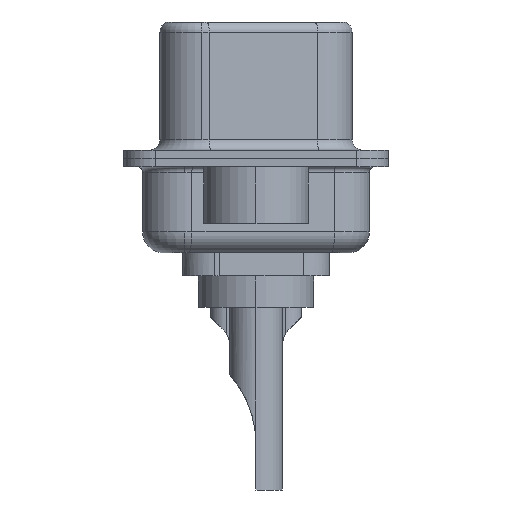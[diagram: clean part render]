
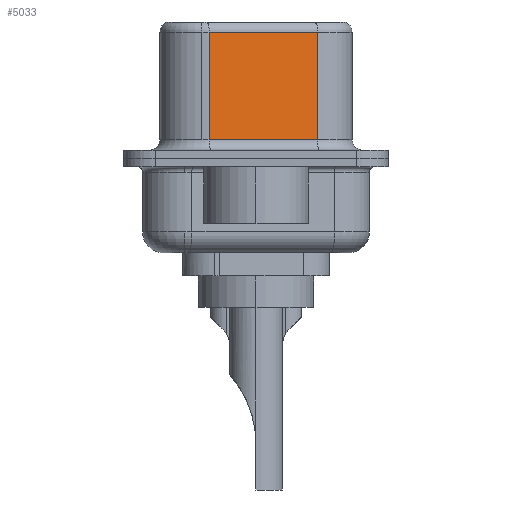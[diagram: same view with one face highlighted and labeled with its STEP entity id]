
A CAD part, left-side view. The second image highlights one B-rep face of the part: STEP entity #5033.
In plain terms, the highlighted planar face has unit normal (-0.985, -0.174, 0).
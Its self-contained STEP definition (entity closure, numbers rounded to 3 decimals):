
#11 = CARTESIAN_POINT ( 'NONE',  ( 4.585, -2.927, 0.9 ) ) ;
#1015 = VERTEX_POINT ( 'NONE', #20164 ) ;
#1697 = AXIS2_PLACEMENT_3D ( 'NONE', #19603, #19473, #19910 ) ;
#2051 = ORIENTED_EDGE ( 'NONE', *, *, #18329, .T. ) ;
#3246 = LINE ( 'NONE', #13953, #20159 ) ;
#4359 = DIRECTION ( 'NONE',  ( 0., 0., -1. ) ) ;
#5033 = ADVANCED_FACE ( 'NONE', ( #6425 ), #19502, .F. ) ;
#5819 = CARTESIAN_POINT ( 'NONE',  ( 4.585, -2.927, 0.9 ) ) ;
#6425 = FACE_OUTER_BOUND ( 'NONE', #9357, .T. ) ;
#6774 = VECTOR ( 'NONE', #16680, 1000. ) ;
#7496 = DIRECTION ( 'NONE',  ( 0.174, -0.985, 0. ) ) ;
#9357 = EDGE_LOOP ( 'NONE', ( #9872, #2051, #13178, #13997 ) ) ;
#9872 = ORIENTED_EDGE ( 'NONE', *, *, #20446, .F. ) ;
#10962 = EDGE_CURVE ( 'NONE', #19362, #16853, #13005, .T. ) ;
#11907 = VERTEX_POINT ( 'NONE', #14026 ) ;
#13005 = LINE ( 'NONE', #5819, #20599 ) ;
#13178 = ORIENTED_EDGE ( 'NONE', *, *, #15770, .T. ) ;
#13647 = CARTESIAN_POINT ( 'NONE',  ( 4.585, -2.927, 6.02 ) ) ;
#13953 = CARTESIAN_POINT ( 'NONE',  ( 3.675, 2.233, 6.52 ) ) ;
#13997 = ORIENTED_EDGE ( 'NONE', *, *, #10962, .T. ) ;
#14026 = CARTESIAN_POINT ( 'NONE',  ( 3.675, 2.233, 6.02 ) ) ;
#15343 = VECTOR ( 'NONE', #4359, 1000. ) ;
#15770 = EDGE_CURVE ( 'NONE', #11907, #19362, #3246, .T. ) ;
#16680 = DIRECTION ( 'NONE',  ( -0.174, 0.985, 0. ) ) ;
#16853 = VERTEX_POINT ( 'NONE', #11 ) ;
#17044 = DIRECTION ( 'NONE',  ( 0., 0., -1. ) ) ;
#18329 = EDGE_CURVE ( 'NONE', #1015, #11907, #19183, .T. ) ;
#18987 = CARTESIAN_POINT ( 'NONE',  ( 4.585, -2.927, 6.52 ) ) ;
#19183 = LINE ( 'NONE', #13647, #6774 ) ;
#19362 = VERTEX_POINT ( 'NONE', #20320 ) ;
#19473 = DIRECTION ( 'NONE',  ( 0.985, 0.174, 0. ) ) ;
#19502 = PLANE ( 'NONE',  #1697 ) ;
#19603 = CARTESIAN_POINT ( 'NONE',  ( 4.585, -2.927, 6.52 ) ) ;
#19689 = LINE ( 'NONE', #18987, #15343 ) ;
#19910 = DIRECTION ( 'NONE',  ( -0.174, 0.985, 0. ) ) ;
#20159 = VECTOR ( 'NONE', #17044, 1000. ) ;
#20164 = CARTESIAN_POINT ( 'NONE',  ( 4.585, -2.927, 6.02 ) ) ;
#20320 = CARTESIAN_POINT ( 'NONE',  ( 3.675, 2.233, 0.9 ) ) ;
#20446 = EDGE_CURVE ( 'NONE', #1015, #16853, #19689, .T. ) ;
#20599 = VECTOR ( 'NONE', #7496, 1000. ) ;
